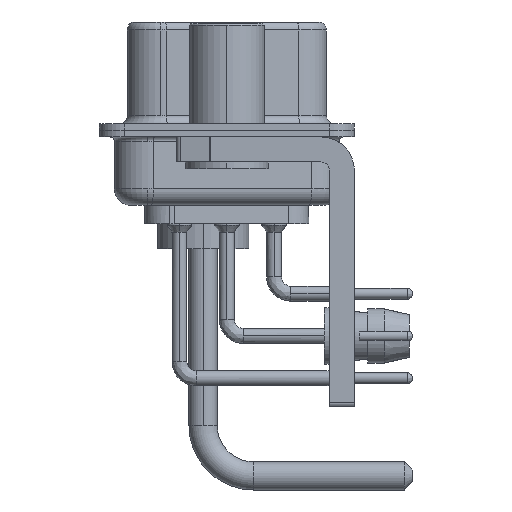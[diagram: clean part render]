
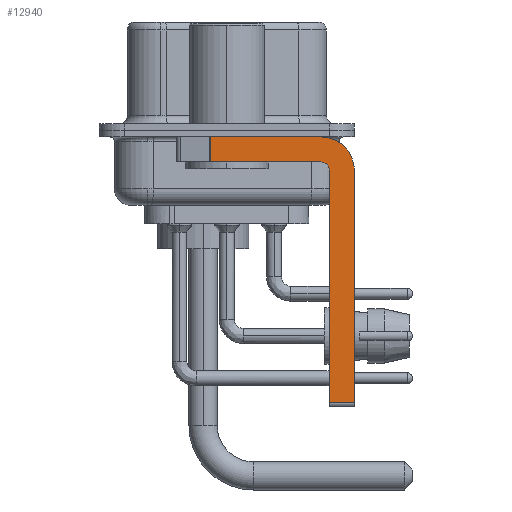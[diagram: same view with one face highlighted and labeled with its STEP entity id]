
A CAD part, left-side view. The second image highlights one B-rep face of the part: STEP entity #12940.
In plain terms, the highlighted planar face has unit normal (-1, 0, 0).
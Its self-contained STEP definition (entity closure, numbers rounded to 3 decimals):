
#1423 = VERTEX_POINT ( 'NONE', #38064 ) ;
#3473 = EDGE_LOOP ( 'NONE', ( #13401, #17029, #24676, #11418, #8523, #10574, #21964, #24257 ) ) ;
#3704 = CARTESIAN_POINT ( 'NONE',  ( -2.9, -5.65, -16.35 ) ) ;
#5156 = FACE_OUTER_BOUND ( 'NONE', #3473, .T. ) ;
#5552 = DIRECTION ( 'NONE',  ( 1., 0., 0. ) ) ;
#6684 = DIRECTION ( 'NONE',  ( 0., 0., 1. ) ) ;
#6821 = DIRECTION ( 'NONE',  ( 0., -1., 0. ) ) ;
#6882 = CARTESIAN_POINT ( 'NONE',  ( -2.9, -6.15, -16.6 ) ) ;
#7124 = VERTEX_POINT ( 'NONE', #9033 ) ;
#8523 = ORIENTED_EDGE ( 'NONE', *, *, #40791, .F. ) ;
#8623 = LINE ( 'NONE', #6882, #26845 ) ;
#9033 = CARTESIAN_POINT ( 'NONE',  ( -2.9, -5.65, -0.4 ) ) ;
#9632 = VERTEX_POINT ( 'NONE', #33688 ) ;
#10471 = CARTESIAN_POINT ( 'NONE',  ( -2.9, -5.65, -1.9 ) ) ;
#10574 = ORIENTED_EDGE ( 'NONE', *, *, #11244, .T. ) ;
#11244 = EDGE_CURVE ( 'NONE', #17126, #1423, #15517, .T. ) ;
#11418 = ORIENTED_EDGE ( 'NONE', *, *, #13575, .F. ) ;
#12685 = AXIS2_PLACEMENT_3D ( 'NONE', #37032, #5552, #27291 ) ;
#12895 = DIRECTION ( 'NONE',  ( -1., 0., 0. ) ) ;
#12932 = CARTESIAN_POINT ( 'NONE',  ( -2.9, -6.15, -16.35 ) ) ;
#12940 = ADVANCED_FACE ( 'NONE', ( #5156 ), #17793, .F. ) ;
#13401 = ORIENTED_EDGE ( 'NONE', *, *, #24035, .F. ) ;
#13563 = CARTESIAN_POINT ( 'NONE',  ( -2.9, 0.978, -1.9 ) ) ;
#13575 = EDGE_CURVE ( 'NONE', #24705, #9632, #28817, .T. ) ;
#14550 = AXIS2_PLACEMENT_3D ( 'NONE', #30024, #33128, #33540 ) ;
#14782 = LINE ( 'NONE', #30500, #15554 ) ;
#15154 = DIRECTION ( 'NONE',  ( 0., -1., 0. ) ) ;
#15517 = LINE ( 'NONE', #3704, #20794 ) ;
#15554 = VECTOR ( 'NONE', #33790, 1000. ) ;
#17029 = ORIENTED_EDGE ( 'NONE', *, *, #22413, .T. ) ;
#17126 = VERTEX_POINT ( 'NONE', #12932 ) ;
#17336 = EDGE_CURVE ( 'NONE', #31169, #1423, #14782, .T. ) ;
#17487 = CARTESIAN_POINT ( 'NONE',  ( -2.9, -6.15, -2.4 ) ) ;
#17793 = PLANE ( 'NONE',  #12685 ) ;
#19600 = AXIS2_PLACEMENT_3D ( 'NONE', #25105, #12895, #6684 ) ;
#19969 = VECTOR ( 'NONE', #35503, 1000. ) ;
#20794 = VECTOR ( 'NONE', #6821, 1000. ) ;
#21964 = ORIENTED_EDGE ( 'NONE', *, *, #17336, .F. ) ;
#22413 = EDGE_CURVE ( 'NONE', #26679, #35445, #39355, .T. ) ;
#22486 = EDGE_CURVE ( 'NONE', #7124, #31169, #29711, .T. ) ;
#24035 = EDGE_CURVE ( 'NONE', #26679, #7124, #27549, .T. ) ;
#24257 = ORIENTED_EDGE ( 'NONE', *, *, #22486, .F. ) ;
#24649 = EDGE_CURVE ( 'NONE', #9632, #35445, #35710, .T. ) ;
#24669 = CARTESIAN_POINT ( 'NONE',  ( -2.9, 0.978, -0.4 ) ) ;
#24676 = ORIENTED_EDGE ( 'NONE', *, *, #24649, .F. ) ;
#24705 = VERTEX_POINT ( 'NONE', #17487 ) ;
#25105 = CARTESIAN_POINT ( 'NONE',  ( -2.9, -5.65, -2.4 ) ) ;
#26679 = VERTEX_POINT ( 'NONE', #24669 ) ;
#26845 = VECTOR ( 'NONE', #30562, 1000. ) ;
#27195 = VECTOR ( 'NONE', #15154, 1000. ) ;
#27291 = DIRECTION ( 'NONE',  ( 0., 0., -1. ) ) ;
#27320 = CARTESIAN_POINT ( 'NONE',  ( -2.9, 0.978, -1.9 ) ) ;
#27549 = LINE ( 'NONE', #40807, #27195 ) ;
#28817 = CIRCLE ( 'NONE', #19600, 0.5 ) ;
#29050 = VECTOR ( 'NONE', #39975, 1000. ) ;
#29711 = CIRCLE ( 'NONE', #14550, 2. ) ;
#30024 = CARTESIAN_POINT ( 'NONE',  ( -2.9, -5.65, -2.4 ) ) ;
#30500 = CARTESIAN_POINT ( 'NONE',  ( -2.9, -7.65, -2.4 ) ) ;
#30562 = DIRECTION ( 'NONE',  ( 0., 0., 1. ) ) ;
#31169 = VERTEX_POINT ( 'NONE', #35846 ) ;
#33128 = DIRECTION ( 'NONE',  ( 1., 0., 0. ) ) ;
#33540 = DIRECTION ( 'NONE',  ( 0., 0., -1. ) ) ;
#33688 = CARTESIAN_POINT ( 'NONE',  ( -2.9, -5.65, -1.9 ) ) ;
#33790 = DIRECTION ( 'NONE',  ( 0., 0., -1. ) ) ;
#35445 = VERTEX_POINT ( 'NONE', #13563 ) ;
#35503 = DIRECTION ( 'NONE',  ( 0., 1., 0. ) ) ;
#35710 = LINE ( 'NONE', #10471, #19969 ) ;
#35846 = CARTESIAN_POINT ( 'NONE',  ( -2.9, -7.65, -2.4 ) ) ;
#37032 = CARTESIAN_POINT ( 'NONE',  ( -2.9, -5.65, -2.4 ) ) ;
#38064 = CARTESIAN_POINT ( 'NONE',  ( -2.9, -7.65, -16.35 ) ) ;
#39355 = LINE ( 'NONE', #27320, #29050 ) ;
#39975 = DIRECTION ( 'NONE',  ( 0., 0., -1. ) ) ;
#40791 = EDGE_CURVE ( 'NONE', #17126, #24705, #8623, .T. ) ;
#40807 = CARTESIAN_POINT ( 'NONE',  ( -2.9, 3., -0.4 ) ) ;
